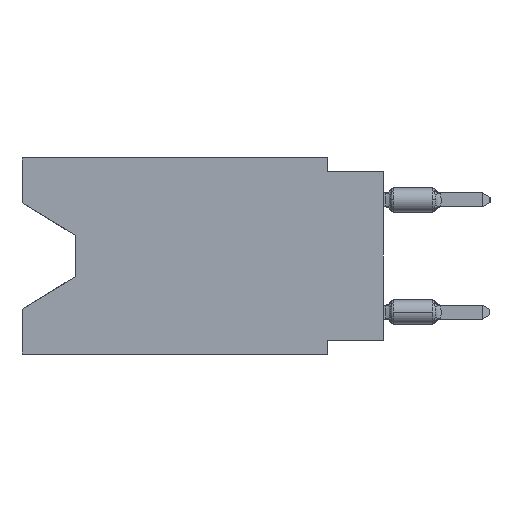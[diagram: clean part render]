
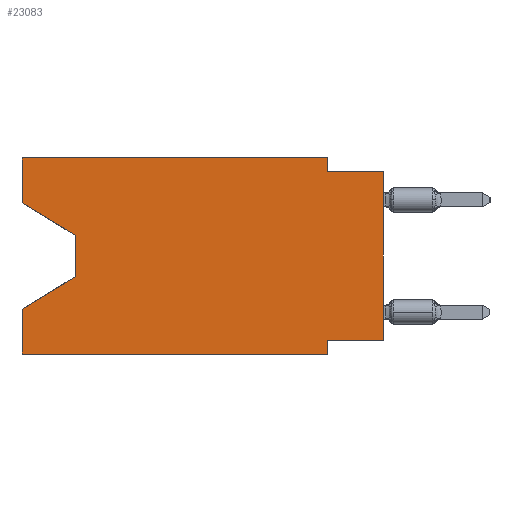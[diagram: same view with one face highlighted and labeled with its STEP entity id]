
A CAD part, left-side view. The second image highlights one B-rep face of the part: STEP entity #23083.
In plain terms, the highlighted planar face has unit normal (-1, 0, 0).
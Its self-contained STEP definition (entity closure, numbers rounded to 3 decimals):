
#377 = EDGE_CURVE ( 'NONE', #29009, #23798, #10678, .T. ) ;
#1090 = CARTESIAN_POINT ( 'NONE',  ( 0., 13.97, -3.505 ) ) ;
#1171 = VECTOR ( 'NONE', #2928, 1000. ) ;
#2195 = LINE ( 'NONE', #33878, #19797 ) ;
#2533 = LINE ( 'NONE', #14365, #39638 ) ;
#2731 = CARTESIAN_POINT ( 'NONE',  ( 0., 2.54, -8.255 ) ) ;
#2878 = EDGE_CURVE ( 'NONE', #14765, #42237, #2533, .T. ) ;
#2928 = DIRECTION ( 'NONE',  ( 0., 1., 0. ) ) ;
#2988 = EDGE_CURVE ( 'NONE', #32069, #33579, #19767, .T. ) ;
#3378 = ORIENTED_EDGE ( 'NONE', *, *, #377, .T. ) ;
#4510 = DIRECTION ( 'NONE',  ( 0., 0., -1. ) ) ;
#4833 = VECTOR ( 'NONE', #36998, 1000. ) ;
#5467 = CARTESIAN_POINT ( 'NONE',  ( 0., 2.54, -0.635 ) ) ;
#5717 = ORIENTED_EDGE ( 'NONE', *, *, #26703, .T. ) ;
#7253 = AXIS2_PLACEMENT_3D ( 'NONE', #16299, #8334, #16041 ) ;
#7512 = ORIENTED_EDGE ( 'NONE', *, *, #40517, .T. ) ;
#8334 = DIRECTION ( 'NONE',  ( 1., 0., 0. ) ) ;
#8575 = FACE_OUTER_BOUND ( 'NONE', #48655, .T. ) ;
#8827 = PLANE ( 'NONE',  #7253 ) ;
#8900 = DIRECTION ( 'NONE',  ( 0., 0., 1. ) ) ;
#10274 = EDGE_CURVE ( 'NONE', #40347, #45024, #2195, .T. ) ;
#10678 = LINE ( 'NONE', #45720, #36983 ) ;
#10832 = CARTESIAN_POINT ( 'NONE',  ( 0., 16.383, -2.038 ) ) ;
#11529 = CARTESIAN_POINT ( 'NONE',  ( 0., 16.383, 0. ) ) ;
#11592 = VECTOR ( 'NONE', #4510, 1000. ) ;
#12073 = ORIENTED_EDGE ( 'NONE', *, *, #17283, .T. ) ;
#14085 = VERTEX_POINT ( 'NONE', #35673 ) ;
#14365 = CARTESIAN_POINT ( 'NONE',  ( 0., 2.54, 0. ) ) ;
#14632 = VERTEX_POINT ( 'NONE', #1090 ) ;
#14765 = VERTEX_POINT ( 'NONE', #37383 ) ;
#14808 = CARTESIAN_POINT ( 'NONE',  ( 0., 16.383, -2.038 ) ) ;
#14821 = DIRECTION ( 'NONE',  ( 0., -1., 0. ) ) ;
#15130 = EDGE_CURVE ( 'NONE', #33579, #14765, #49887, .T. ) ;
#15190 = VECTOR ( 'NONE', #8900, 1000. ) ;
#16006 = LINE ( 'NONE', #28618, #19453 ) ;
#16041 = DIRECTION ( 'NONE',  ( 0., 0., -1. ) ) ;
#16299 = CARTESIAN_POINT ( 'NONE',  ( 0., 16.383, 0. ) ) ;
#16371 = CARTESIAN_POINT ( 'NONE',  ( 0., 0., 0. ) ) ;
#16418 = EDGE_CURVE ( 'NONE', #42032, #23798, #16006, .T. ) ;
#17283 = EDGE_CURVE ( 'NONE', #42032, #45024, #33628, .T. ) ;
#18061 = ORIENTED_EDGE ( 'NONE', *, *, #29633, .F. ) ;
#19445 = LINE ( 'NONE', #39801, #11592 ) ;
#19453 = VECTOR ( 'NONE', #27609, 1000. ) ;
#19587 = ORIENTED_EDGE ( 'NONE', *, *, #2878, .F. ) ;
#19654 = LINE ( 'NONE', #50862, #39139 ) ;
#19767 = LINE ( 'NONE', #11529, #25638 ) ;
#19797 = VECTOR ( 'NONE', #22514, 1000. ) ;
#20236 = LINE ( 'NONE', #16371, #15190 ) ;
#21017 = CARTESIAN_POINT ( 'NONE',  ( 0., 16.383, -8.89 ) ) ;
#21054 = ORIENTED_EDGE ( 'NONE', *, *, #10274, .F. ) ;
#22009 = DIRECTION ( 'NONE',  ( 0., 0.855, -0.519 ) ) ;
#22514 = DIRECTION ( 'NONE',  ( 0., 0., -1. ) ) ;
#22862 = CARTESIAN_POINT ( 'NONE',  ( 0., 16.383, -6.852 ) ) ;
#23035 = DIRECTION ( 'NONE',  ( 0., -0.855, -0.519 ) ) ;
#23083 = ADVANCED_FACE ( 'NONE', ( #8575 ), #8827, .F. ) ;
#23798 = VERTEX_POINT ( 'NONE', #22862 ) ;
#24031 = EDGE_CURVE ( 'NONE', #43003, #40347, #25088, .T. ) ;
#25088 = LINE ( 'NONE', #29470, #1171 ) ;
#25638 = VECTOR ( 'NONE', #35737, 1000. ) ;
#26351 = DIRECTION ( 'NONE',  ( 0., -1., 0. ) ) ;
#26457 = DIRECTION ( 'NONE',  ( 0., 0., -1. ) ) ;
#26497 = ORIENTED_EDGE ( 'NONE', *, *, #24031, .F. ) ;
#26703 = EDGE_CURVE ( 'NONE', #43003, #14085, #20236, .T. ) ;
#26725 = ORIENTED_EDGE ( 'NONE', *, *, #15130, .F. ) ;
#26983 = VECTOR ( 'NONE', #23035, 1000. ) ;
#27609 = DIRECTION ( 'NONE',  ( 0., 0., 1. ) ) ;
#28196 = CARTESIAN_POINT ( 'NONE',  ( 0., 0., -8.255 ) ) ;
#28280 = CARTESIAN_POINT ( 'NONE',  ( 0., 2.54, -8.89 ) ) ;
#28618 = CARTESIAN_POINT ( 'NONE',  ( 0., 16.383, 0. ) ) ;
#29009 = VERTEX_POINT ( 'NONE', #48878 ) ;
#29470 = CARTESIAN_POINT ( 'NONE',  ( 0., 0., -8.255 ) ) ;
#29633 = EDGE_CURVE ( 'NONE', #42237, #14085, #19654, .T. ) ;
#30288 = CARTESIAN_POINT ( 'NONE',  ( 0., 16.383, -8.89 ) ) ;
#31714 = VECTOR ( 'NONE', #14821, 1000. ) ;
#32069 = VERTEX_POINT ( 'NONE', #10832 ) ;
#32814 = ORIENTED_EDGE ( 'NONE', *, *, #49015, .T. ) ;
#33579 = VERTEX_POINT ( 'NONE', #37336 ) ;
#33628 = LINE ( 'NONE', #21017, #4833 ) ;
#33878 = CARTESIAN_POINT ( 'NONE',  ( 0., 2.54, -8.89 ) ) ;
#34384 = LINE ( 'NONE', #14808, #26983 ) ;
#35673 = CARTESIAN_POINT ( 'NONE',  ( 0., 0., -0.635 ) ) ;
#35737 = DIRECTION ( 'NONE',  ( 0., 0., 1. ) ) ;
#36983 = VECTOR ( 'NONE', #22009, 1000. ) ;
#36998 = DIRECTION ( 'NONE',  ( 0., -1., 0. ) ) ;
#37336 = CARTESIAN_POINT ( 'NONE',  ( 0., 16.383, 0. ) ) ;
#37383 = CARTESIAN_POINT ( 'NONE',  ( 0., 2.54, 0. ) ) ;
#39139 = VECTOR ( 'NONE', #26351, 1000. ) ;
#39638 = VECTOR ( 'NONE', #26457, 1000. ) ;
#39801 = CARTESIAN_POINT ( 'NONE',  ( 0., 13.97, -3.505 ) ) ;
#40347 = VERTEX_POINT ( 'NONE', #2731 ) ;
#40517 = EDGE_CURVE ( 'NONE', #14632, #29009, #19445, .T. ) ;
#42032 = VERTEX_POINT ( 'NONE', #30288 ) ;
#42237 = VERTEX_POINT ( 'NONE', #5467 ) ;
#42905 = ORIENTED_EDGE ( 'NONE', *, *, #2988, .F. ) ;
#43003 = VERTEX_POINT ( 'NONE', #28196 ) ;
#45024 = VERTEX_POINT ( 'NONE', #28280 ) ;
#45720 = CARTESIAN_POINT ( 'NONE',  ( 0., 13.97, -5.385 ) ) ;
#46008 = CARTESIAN_POINT ( 'NONE',  ( 0., 16.383, 0. ) ) ;
#48655 = EDGE_LOOP ( 'NONE', ( #32814, #7512, #3378, #48775, #12073, #21054, #26497, #5717, #18061, #19587, #26725, #42905 ) ) ;
#48775 = ORIENTED_EDGE ( 'NONE', *, *, #16418, .F. ) ;
#48878 = CARTESIAN_POINT ( 'NONE',  ( 0., 13.97, -5.385 ) ) ;
#49015 = EDGE_CURVE ( 'NONE', #32069, #14632, #34384, .T. ) ;
#49887 = LINE ( 'NONE', #46008, #31714 ) ;
#50862 = CARTESIAN_POINT ( 'NONE',  ( 0., 0., -0.635 ) ) ;
